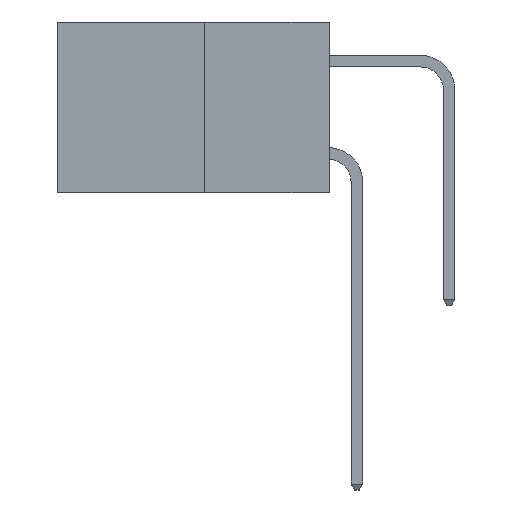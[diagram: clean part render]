
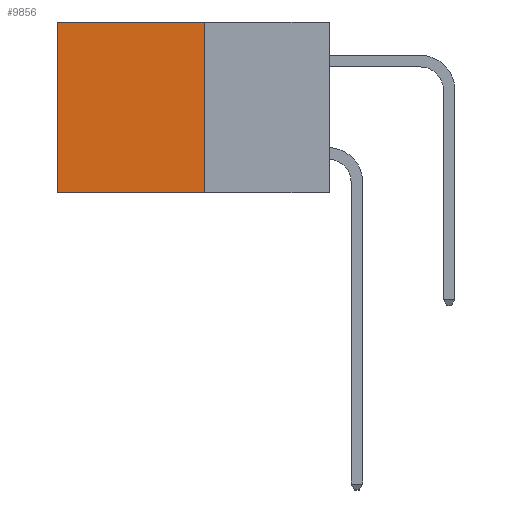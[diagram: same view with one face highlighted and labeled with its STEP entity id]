
A CAD part, left-side view. The second image highlights one B-rep face of the part: STEP entity #9856.
In plain terms, the highlighted planar face has unit normal (-1, 0, 0).
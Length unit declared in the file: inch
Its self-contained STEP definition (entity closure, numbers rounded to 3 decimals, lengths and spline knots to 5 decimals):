
#16 = VERTEX_POINT ( 'NONE', #6380 ) ;
#460 = LINE ( 'NONE', #4078, #3219 ) ;
#919 = VERTEX_POINT ( 'NONE', #9884 ) ;
#1738 = AXIS2_PLACEMENT_3D ( 'NONE', #10395, #11374, #5486 ) ;
#1796 = EDGE_CURVE ( 'NONE', #919, #16, #460, .T. ) ;
#2313 = ORIENTED_EDGE ( 'NONE', *, *, #2680, .F. ) ;
#2459 = CARTESIAN_POINT ( 'NONE',  ( 0.277, 0.59, 0. ) ) ;
#2680 = EDGE_CURVE ( 'NONE', #9896, #919, #4421, .T. ) ;
#3123 = ORIENTED_EDGE ( 'NONE', *, *, #1796, .F. ) ;
#3219 = VECTOR ( 'NONE', #4061, 39.37008 ) ;
#3736 = VECTOR ( 'NONE', #11874, 39.37008 ) ;
#4061 = DIRECTION ( 'NONE',  ( 0., 1., 0. ) ) ;
#4078 = CARTESIAN_POINT ( 'NONE',  ( 0.277, 0.27, -0.37 ) ) ;
#4359 = PLANE ( 'NONE',  #1738 ) ;
#4421 = LINE ( 'NONE', #5289, #9505 ) ;
#4786 = VECTOR ( 'NONE', #8651, 39.37008 ) ;
#5141 = LINE ( 'NONE', #9627, #4786 ) ;
#5201 = DIRECTION ( 'NONE',  ( 0., 0., -1. ) ) ;
#5289 = CARTESIAN_POINT ( 'NONE',  ( 0.277, 0.27, -0.37 ) ) ;
#5486 = DIRECTION ( 'NONE',  ( 0., 0., -1. ) ) ;
#5830 = EDGE_LOOP ( 'NONE', ( #6179, #3123, #2313, #6025 ) ) ;
#6025 = ORIENTED_EDGE ( 'NONE', *, *, #6129, .T. ) ;
#6129 = EDGE_CURVE ( 'NONE', #9896, #12433, #9234, .T. ) ;
#6179 = ORIENTED_EDGE ( 'NONE', *, *, #6336, .T. ) ;
#6336 = EDGE_CURVE ( 'NONE', #12433, #16, #5141, .T. ) ;
#6380 = CARTESIAN_POINT ( 'NONE',  ( 0.277, 0.59, -0.37 ) ) ;
#8503 = CARTESIAN_POINT ( 'NONE',  ( 0.277, 0.27, 0. ) ) ;
#8651 = DIRECTION ( 'NONE',  ( 0., 0., -1. ) ) ;
#9234 = LINE ( 'NONE', #10894, #3736 ) ;
#9487 = FACE_OUTER_BOUND ( 'NONE', #5830, .T. ) ;
#9505 = VECTOR ( 'NONE', #5201, 39.37008 ) ;
#9627 = CARTESIAN_POINT ( 'NONE',  ( 0.277, 0.59, -0.37 ) ) ;
#9856 = ADVANCED_FACE ( 'NONE', ( #9487 ), #4359, .F. ) ;
#9884 = CARTESIAN_POINT ( 'NONE',  ( 0.277, 0.27, -0.37 ) ) ;
#9896 = VERTEX_POINT ( 'NONE', #8503 ) ;
#10395 = CARTESIAN_POINT ( 'NONE',  ( 0.277, 0.27, -0.37 ) ) ;
#10894 = CARTESIAN_POINT ( 'NONE',  ( 0.277, 0.27, 0. ) ) ;
#11374 = DIRECTION ( 'NONE',  ( 1., 0., 0. ) ) ;
#11874 = DIRECTION ( 'NONE',  ( 0., 1., 0. ) ) ;
#12433 = VERTEX_POINT ( 'NONE', #2459 ) ;
